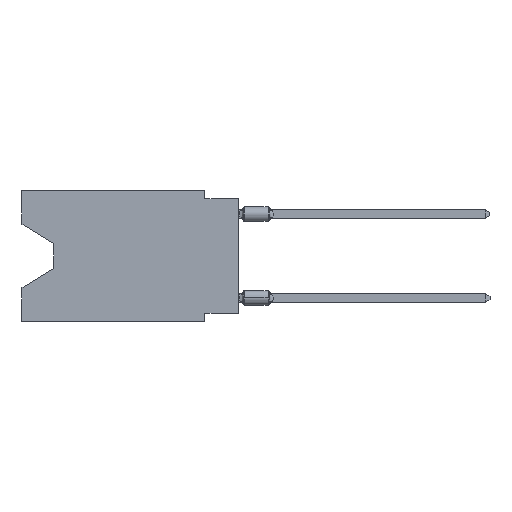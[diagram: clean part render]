
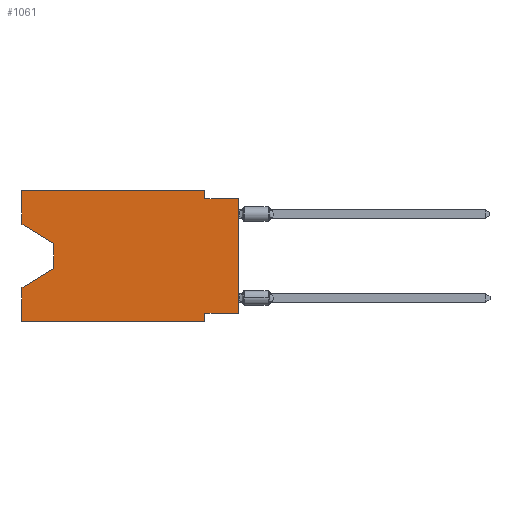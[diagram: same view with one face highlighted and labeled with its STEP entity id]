
A CAD part, left-side view. The second image highlights one B-rep face of the part: STEP entity #1061.
In plain terms, the highlighted planar face has unit normal (-1, 0, 0).
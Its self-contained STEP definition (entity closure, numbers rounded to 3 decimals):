
#535 = DIRECTION ( 'NONE',  ( 1., 0., 0. ) ) ;
#591 = EDGE_CURVE ( 'NONE', #6048, #2589, #11264, .T. ) ;
#823 = CARTESIAN_POINT ( 'NONE',  ( 0., 13.97, -5.893 ) ) ;
#1061 = ADVANCED_FACE ( 'NONE', ( #3471 ), #3376, .F. ) ;
#1239 = DIRECTION ( 'NONE',  ( 0., -1., 0. ) ) ;
#1704 = DIRECTION ( 'NONE',  ( 0., 0., -1. ) ) ;
#1726 = DIRECTION ( 'NONE',  ( 0., 0., 1. ) ) ;
#1812 = CARTESIAN_POINT ( 'NONE',  ( 0., 16.383, -9.906 ) ) ;
#1910 = ORIENTED_EDGE ( 'NONE', *, *, #16609, .F. ) ;
#2515 = VERTEX_POINT ( 'NONE', #19941 ) ;
#2589 = VERTEX_POINT ( 'NONE', #3154 ) ;
#2661 = VECTOR ( 'NONE', #11084, 1000. ) ;
#2735 = ORIENTED_EDGE ( 'NONE', *, *, #591, .T. ) ;
#2778 = CARTESIAN_POINT ( 'NONE',  ( 0., 16.383, -9.906 ) ) ;
#2986 = VERTEX_POINT ( 'NONE', #9396 ) ;
#3154 = CARTESIAN_POINT ( 'NONE',  ( 0., 0., -0.635 ) ) ;
#3241 = VERTEX_POINT ( 'NONE', #19993 ) ;
#3376 = PLANE ( 'NONE',  #19020 ) ;
#3411 = CARTESIAN_POINT ( 'NONE',  ( 0., 0., -9.271 ) ) ;
#3471 = FACE_OUTER_BOUND ( 'NONE', #6083, .T. ) ;
#3804 = VECTOR ( 'NONE', #6991, 1000. ) ;
#4446 = CARTESIAN_POINT ( 'NONE',  ( 0., 2.54, -9.906 ) ) ;
#4853 = DIRECTION ( 'NONE',  ( 0., -1., 0. ) ) ;
#4895 = DIRECTION ( 'NONE',  ( 0., 0., -1. ) ) ;
#4935 = LINE ( 'NONE', #5040, #2661 ) ;
#5040 = CARTESIAN_POINT ( 'NONE',  ( 0., 13.97, -4.013 ) ) ;
#5053 = LINE ( 'NONE', #11195, #18832 ) ;
#5080 = CARTESIAN_POINT ( 'NONE',  ( 0., 2.54, 0. ) ) ;
#5211 = EDGE_CURVE ( 'NONE', #5757, #2589, #17618, .T. ) ;
#5348 = DIRECTION ( 'NONE',  ( 0., 0., -1. ) ) ;
#5507 = DIRECTION ( 'NONE',  ( 0., -1., 0. ) ) ;
#5757 = VERTEX_POINT ( 'NONE', #15569 ) ;
#6048 = VERTEX_POINT ( 'NONE', #15211 ) ;
#6083 = EDGE_LOOP ( 'NONE', ( #16292, #10221, #11626, #12789, #18971, #14033, #12550, #2735, #16972, #18631, #6451, #1910 ) ) ;
#6420 = EDGE_CURVE ( 'NONE', #16578, #6683, #13077, .T. ) ;
#6451 = ORIENTED_EDGE ( 'NONE', *, *, #6420, .F. ) ;
#6525 = CARTESIAN_POINT ( 'NONE',  ( 0., 0., 0. ) ) ;
#6666 = VERTEX_POINT ( 'NONE', #19098 ) ;
#6683 = VERTEX_POINT ( 'NONE', #5080 ) ;
#6991 = DIRECTION ( 'NONE',  ( 0., 0.855, -0.519 ) ) ;
#7012 = CARTESIAN_POINT ( 'NONE',  ( 0., 2.54, -9.271 ) ) ;
#7514 = LINE ( 'NONE', #13794, #15354 ) ;
#7940 = CARTESIAN_POINT ( 'NONE',  ( 0., 16.383, 0. ) ) ;
#8085 = VECTOR ( 'NONE', #1726, 1000. ) ;
#8114 = CARTESIAN_POINT ( 'NONE',  ( 0., 16.383, 0. ) ) ;
#8722 = CARTESIAN_POINT ( 'NONE',  ( 0., 16.383, 0. ) ) ;
#8865 = VECTOR ( 'NONE', #9359, 1000. ) ;
#9172 = VERTEX_POINT ( 'NONE', #2778 ) ;
#9359 = DIRECTION ( 'NONE',  ( 0., 0., 1. ) ) ;
#9396 = CARTESIAN_POINT ( 'NONE',  ( 0., 13.97, -5.893 ) ) ;
#9793 = LINE ( 'NONE', #17190, #8085 ) ;
#9934 = CARTESIAN_POINT ( 'NONE',  ( 0., 0., -0.635 ) ) ;
#10221 = ORIENTED_EDGE ( 'NONE', *, *, #14944, .T. ) ;
#10968 = LINE ( 'NONE', #7940, #8865 ) ;
#11084 = DIRECTION ( 'NONE',  ( 0., 0., -1. ) ) ;
#11195 = CARTESIAN_POINT ( 'NONE',  ( 0., 2.54, 0. ) ) ;
#11264 = LINE ( 'NONE', #6525, #18412 ) ;
#11482 = VECTOR ( 'NONE', #4853, 1000. ) ;
#11626 = ORIENTED_EDGE ( 'NONE', *, *, #11696, .T. ) ;
#11696 = EDGE_CURVE ( 'NONE', #2986, #14039, #14681, .T. ) ;
#12076 = VECTOR ( 'NONE', #1239, 1000. ) ;
#12119 = LINE ( 'NONE', #4446, #15039 ) ;
#12550 = ORIENTED_EDGE ( 'NONE', *, *, #14935, .F. ) ;
#12789 = ORIENTED_EDGE ( 'NONE', *, *, #19543, .F. ) ;
#12810 = LINE ( 'NONE', #3411, #17506 ) ;
#13077 = LINE ( 'NONE', #8722, #12076 ) ;
#13794 = CARTESIAN_POINT ( 'NONE',  ( 0., 16.383, -2.546 ) ) ;
#13912 = CARTESIAN_POINT ( 'NONE',  ( 0., 16.383, 0. ) ) ;
#14033 = ORIENTED_EDGE ( 'NONE', *, *, #17791, .F. ) ;
#14039 = VERTEX_POINT ( 'NONE', #18456 ) ;
#14681 = LINE ( 'NONE', #823, #3804 ) ;
#14935 = EDGE_CURVE ( 'NONE', #6048, #18916, #12810, .T. ) ;
#14944 = EDGE_CURVE ( 'NONE', #3241, #2986, #4935, .T. ) ;
#15039 = VECTOR ( 'NONE', #1704, 1000. ) ;
#15211 = CARTESIAN_POINT ( 'NONE',  ( 0., 0., -9.271 ) ) ;
#15354 = VECTOR ( 'NONE', #16511, 1000. ) ;
#15451 = DIRECTION ( 'NONE',  ( 0., 1., 0. ) ) ;
#15569 = CARTESIAN_POINT ( 'NONE',  ( 0., 2.54, -0.635 ) ) ;
#16292 = ORIENTED_EDGE ( 'NONE', *, *, #16899, .T. ) ;
#16511 = DIRECTION ( 'NONE',  ( 0., -0.855, -0.519 ) ) ;
#16578 = VERTEX_POINT ( 'NONE', #13912 ) ;
#16609 = EDGE_CURVE ( 'NONE', #2515, #16578, #10968, .T. ) ;
#16899 = EDGE_CURVE ( 'NONE', #2515, #3241, #7514, .T. ) ;
#16972 = ORIENTED_EDGE ( 'NONE', *, *, #5211, .F. ) ;
#17190 = CARTESIAN_POINT ( 'NONE',  ( 0., 16.383, 0. ) ) ;
#17437 = DIRECTION ( 'NONE',  ( 0., 0., 1. ) ) ;
#17506 = VECTOR ( 'NONE', #15451, 1000. ) ;
#17618 = LINE ( 'NONE', #9934, #17838 ) ;
#17765 = EDGE_CURVE ( 'NONE', #9172, #6666, #18385, .T. ) ;
#17791 = EDGE_CURVE ( 'NONE', #18916, #6666, #12119, .T. ) ;
#17838 = VECTOR ( 'NONE', #5507, 1000. ) ;
#17967 = EDGE_CURVE ( 'NONE', #6683, #5757, #5053, .T. ) ;
#18385 = LINE ( 'NONE', #1812, #11482 ) ;
#18412 = VECTOR ( 'NONE', #17437, 1000. ) ;
#18456 = CARTESIAN_POINT ( 'NONE',  ( 0., 16.383, -7.36 ) ) ;
#18631 = ORIENTED_EDGE ( 'NONE', *, *, #17967, .F. ) ;
#18832 = VECTOR ( 'NONE', #5348, 1000. ) ;
#18916 = VERTEX_POINT ( 'NONE', #7012 ) ;
#18971 = ORIENTED_EDGE ( 'NONE', *, *, #17765, .T. ) ;
#19020 = AXIS2_PLACEMENT_3D ( 'NONE', #8114, #535, #4895 ) ;
#19098 = CARTESIAN_POINT ( 'NONE',  ( 0., 2.54, -9.906 ) ) ;
#19543 = EDGE_CURVE ( 'NONE', #9172, #14039, #9793, .T. ) ;
#19941 = CARTESIAN_POINT ( 'NONE',  ( 0., 16.383, -2.546 ) ) ;
#19993 = CARTESIAN_POINT ( 'NONE',  ( 0., 13.97, -4.013 ) ) ;
